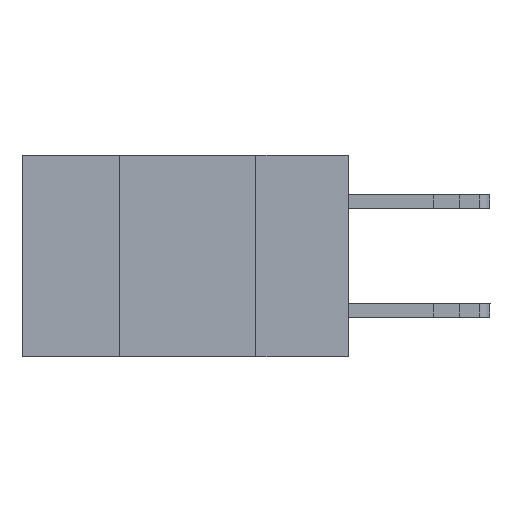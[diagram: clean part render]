
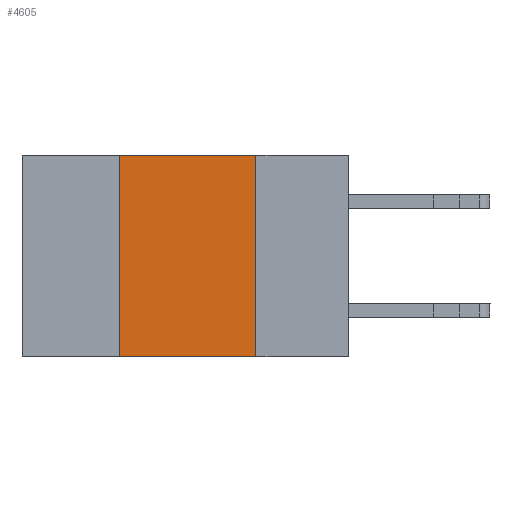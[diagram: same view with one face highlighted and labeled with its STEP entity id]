
A CAD part, left-side view. The second image highlights one B-rep face of the part: STEP entity #4605.
In plain terms, the highlighted planar face has unit normal (-1, 0, 0).
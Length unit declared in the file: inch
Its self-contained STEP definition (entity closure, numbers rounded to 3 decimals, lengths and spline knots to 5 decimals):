
#434 = CARTESIAN_POINT ( 'NONE',  ( 0., 0.42, -0.37 ) ) ;
#676 = VERTEX_POINT ( 'NONE', #434 ) ;
#1046 = AXIS2_PLACEMENT_3D ( 'NONE', #1431, #1301, #1287 ) ;
#1287 = DIRECTION ( 'NONE',  ( 0., 0., -1. ) ) ;
#1301 = DIRECTION ( 'NONE',  ( 1., 0., 0. ) ) ;
#1365 = PLANE ( 'NONE',  #1046 ) ;
#1431 = CARTESIAN_POINT ( 'NONE',  ( 0., 0.6, 0. ) ) ;
#1745 = CARTESIAN_POINT ( 'NONE',  ( 0., 0.42, 0. ) ) ;
#1873 = VECTOR ( 'NONE', #10197, 39.37008 ) ;
#2011 = LINE ( 'NONE', #2255, #14650 ) ;
#2255 = CARTESIAN_POINT ( 'NONE',  ( 0., 0.17, -0.37 ) ) ;
#2508 = VERTEX_POINT ( 'NONE', #7212 ) ;
#2892 = VECTOR ( 'NONE', #5213, 39.37008 ) ;
#3277 = LINE ( 'NONE', #11100, #2892 ) ;
#3395 = FACE_OUTER_BOUND ( 'NONE', #6932, .T. ) ;
#3538 = DIRECTION ( 'NONE',  ( 0., 0., -1. ) ) ;
#4187 = CARTESIAN_POINT ( 'NONE',  ( 0., 0.42, -0.37 ) ) ;
#4605 = ADVANCED_FACE ( 'NONE', ( #3395 ), #1365, .F. ) ;
#5213 = DIRECTION ( 'NONE',  ( 0., -1., 0. ) ) ;
#5227 = LINE ( 'NONE', #4187, #1873 ) ;
#5786 = ORIENTED_EDGE ( 'NONE', *, *, #6575, .T. ) ;
#5955 = CARTESIAN_POINT ( 'NONE',  ( 0., 0.17, 0. ) ) ;
#6575 = EDGE_CURVE ( 'NONE', #676, #2508, #3277, .T. ) ;
#6673 = ORIENTED_EDGE ( 'NONE', *, *, #7338, .F. ) ;
#6728 = ORIENTED_EDGE ( 'NONE', *, *, #8933, .F. ) ;
#6791 = VERTEX_POINT ( 'NONE', #1745 ) ;
#6928 = LINE ( 'NONE', #8032, #10029 ) ;
#6932 = EDGE_LOOP ( 'NONE', ( #6728, #9788, #6673, #5786 ) ) ;
#7212 = CARTESIAN_POINT ( 'NONE',  ( 0., 0.17, -0.37 ) ) ;
#7338 = EDGE_CURVE ( 'NONE', #676, #6791, #5227, .T. ) ;
#8032 = CARTESIAN_POINT ( 'NONE',  ( 0., 0.6, 0. ) ) ;
#8124 = EDGE_CURVE ( 'NONE', #6791, #11107, #6928, .T. ) ;
#8933 = EDGE_CURVE ( 'NONE', #11107, #2508, #2011, .T. ) ;
#9788 = ORIENTED_EDGE ( 'NONE', *, *, #8124, .F. ) ;
#10029 = VECTOR ( 'NONE', #13792, 39.37008 ) ;
#10197 = DIRECTION ( 'NONE',  ( 0., 0., 1. ) ) ;
#11100 = CARTESIAN_POINT ( 'NONE',  ( 0., 0.6, -0.37 ) ) ;
#11107 = VERTEX_POINT ( 'NONE', #5955 ) ;
#13792 = DIRECTION ( 'NONE',  ( 0., -1., 0. ) ) ;
#14650 = VECTOR ( 'NONE', #3538, 39.37008 ) ;
